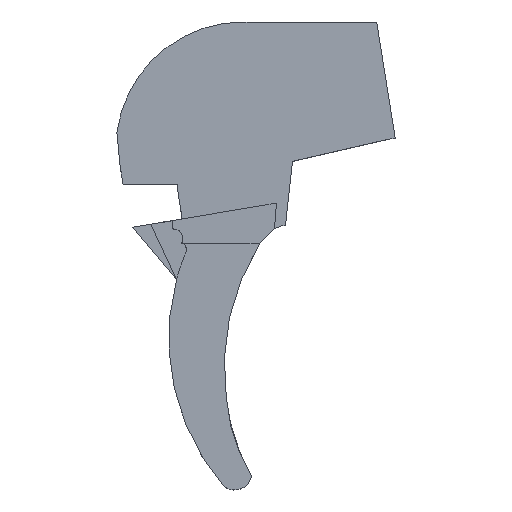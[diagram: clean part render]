
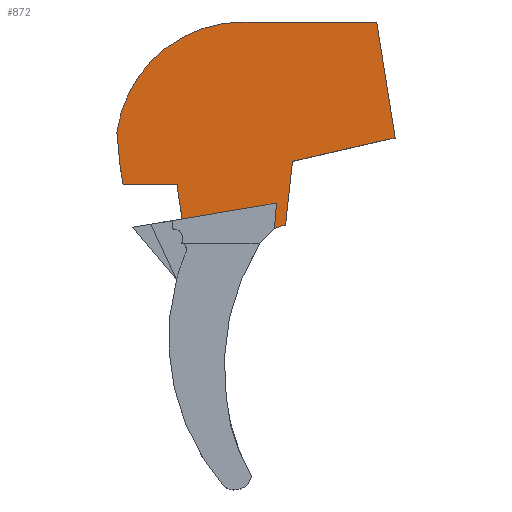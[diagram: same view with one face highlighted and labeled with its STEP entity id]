
A CAD part, top view. The second image highlights one B-rep face of the part: STEP entity #872.
In plain terms, the highlighted planar face has unit normal (0, 0, 1).
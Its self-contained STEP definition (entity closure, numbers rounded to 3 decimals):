
#65=PLANE('',#943);
#100=FACE_OUTER_BOUND('',#148,.T.);
#148=EDGE_LOOP('',(#631,#632,#633,#634,#635,#636,#637,#638,#639,#640,#641,
#642,#643,#644,#645,#646,#647));
#195=LINE('',#1198,#273);
#201=LINE('',#1215,#279);
#218=LINE('',#1272,#296);
#219=LINE('',#1274,#297);
#220=LINE('',#1276,#298);
#221=LINE('',#1277,#299);
#222=LINE('',#1279,#300);
#223=LINE('',#1281,#301);
#224=LINE('',#1283,#302);
#225=LINE('',#1285,#303);
#226=LINE('',#1287,#304);
#227=LINE('',#1289,#305);
#228=LINE('',#1291,#306);
#229=LINE('',#1293,#307);
#230=LINE('',#1294,#308);
#273=VECTOR('',#1000,10.);
#279=VECTOR('',#1014,10.);
#296=VECTOR('',#1045,10.);
#297=VECTOR('',#1046,10.);
#298=VECTOR('',#1047,10.);
#299=VECTOR('',#1048,10.);
#300=VECTOR('',#1049,10.);
#301=VECTOR('',#1050,10.);
#302=VECTOR('',#1051,10.);
#303=VECTOR('',#1052,10.);
#304=VECTOR('',#1053,10.);
#305=VECTOR('',#1054,10.);
#306=VECTOR('',#1055,10.);
#307=VECTOR('',#1056,10.);
#308=VECTOR('',#1057,10.);
#349=CIRCLE('',#930,12.007);
#352=CIRCLE('',#935,3.);
#365=VERTEX_POINT('',#1188);
#366=VERTEX_POINT('',#1189);
#369=VERTEX_POINT('',#1197);
#372=VERTEX_POINT('',#1205);
#375=VERTEX_POINT('',#1212);
#376=VERTEX_POINT('',#1214);
#397=VERTEX_POINT('',#1271);
#398=VERTEX_POINT('',#1273);
#399=VERTEX_POINT('',#1275);
#400=VERTEX_POINT('',#1278);
#401=VERTEX_POINT('',#1280);
#402=VERTEX_POINT('',#1282);
#403=VERTEX_POINT('',#1284);
#404=VERTEX_POINT('',#1286);
#405=VERTEX_POINT('',#1288);
#406=VERTEX_POINT('',#1290);
#407=VERTEX_POINT('',#1292);
#455=EDGE_CURVE('',#365,#366,#349,.T.);
#459=EDGE_CURVE('',#369,#366,#195,.T.);
#464=EDGE_CURVE('',#372,#369,#352,.T.);
#467=EDGE_CURVE('',#376,#375,#201,.T.);
#491=EDGE_CURVE('',#375,#397,#218,.T.);
#492=EDGE_CURVE('',#397,#398,#219,.T.);
#493=EDGE_CURVE('',#398,#399,#220,.T.);
#494=EDGE_CURVE('',#399,#365,#221,.T.);
#495=EDGE_CURVE('',#372,#400,#222,.T.);
#496=EDGE_CURVE('',#400,#401,#223,.T.);
#497=EDGE_CURVE('',#401,#402,#224,.T.);
#498=EDGE_CURVE('',#402,#403,#225,.T.);
#499=EDGE_CURVE('',#404,#403,#226,.T.);
#500=EDGE_CURVE('',#405,#404,#227,.T.);
#501=EDGE_CURVE('',#406,#405,#228,.T.);
#502=EDGE_CURVE('',#406,#407,#229,.T.);
#503=EDGE_CURVE('',#407,#376,#230,.T.);
#631=ORIENTED_EDGE('',*,*,#467,.T.);
#632=ORIENTED_EDGE('',*,*,#491,.T.);
#633=ORIENTED_EDGE('',*,*,#492,.T.);
#634=ORIENTED_EDGE('',*,*,#493,.T.);
#635=ORIENTED_EDGE('',*,*,#494,.T.);
#636=ORIENTED_EDGE('',*,*,#455,.T.);
#637=ORIENTED_EDGE('',*,*,#459,.F.);
#638=ORIENTED_EDGE('',*,*,#464,.F.);
#639=ORIENTED_EDGE('',*,*,#495,.T.);
#640=ORIENTED_EDGE('',*,*,#496,.T.);
#641=ORIENTED_EDGE('',*,*,#497,.T.);
#642=ORIENTED_EDGE('',*,*,#498,.T.);
#643=ORIENTED_EDGE('',*,*,#499,.F.);
#644=ORIENTED_EDGE('',*,*,#500,.F.);
#645=ORIENTED_EDGE('',*,*,#501,.F.);
#646=ORIENTED_EDGE('',*,*,#502,.T.);
#647=ORIENTED_EDGE('',*,*,#503,.T.);
#872=ADVANCED_FACE('',(#100),#65,.T.);
#930=AXIS2_PLACEMENT_3D('',#1190,#992,#993);
#935=AXIS2_PLACEMENT_3D('',#1207,#1008,#1009);
#943=AXIS2_PLACEMENT_3D('',#1270,#1043,#1044);
#992=DIRECTION('center_axis',(0.,0.,
1.));
#993=DIRECTION('ref_axis',(0.,1.,0.));
#1000=DIRECTION('',(-0.094,0.996,0.));
#1008=DIRECTION('center_axis',(0.,0.,
-1.));
#1009=DIRECTION('ref_axis',(-0.809,0.588,0.));
#1014=DIRECTION('',(0.108,0.994,0.));
#1043=DIRECTION('center_axis',(0.,0.,
1.));
#1044=DIRECTION('ref_axis',(0.988,0.156,0.));
#1045=DIRECTION('',(0.975,0.224,0.));
#1046=DIRECTION('',(0.982,0.191,0.));
#1047=DIRECTION('',(-0.156,0.988,0.));
#1048=DIRECTION('',(-1.,0.,0.));
#1049=DIRECTION('',(0.156,-0.988,0.));
#1050=DIRECTION('',(1.,0.,0.));
#1051=DIRECTION('',(0.,-1.,0.));
#1052=DIRECTION('',(0.156,-0.988,0.));
#1053=DIRECTION('',(-0.986,-0.166,0.));
#1054=DIRECTION('',(-0.986,-0.166,0.));
#1055=DIRECTION('',(0.078,0.997,0.));
#1056=DIRECTION('',(0.928,0.373,0.));
#1057=DIRECTION('',(1.,0.,0.));
#1188=CARTESIAN_POINT('',(42.355,145.835,-19.588));
#1189=CARTESIAN_POINT('',(30.449,135.386,-19.588));
#1190=CARTESIAN_POINT('Origin',(42.355,133.828,-19.588));
#1197=CARTESIAN_POINT('',(30.716,132.546,-19.588));
#1198=CARTESIAN_POINT('',(30.539,134.435,-19.588));
#1205=CARTESIAN_POINT('',(30.74,132.357,-19.588));
#1207=CARTESIAN_POINT('Origin',(33.703,132.827,-19.588));
#1212=CARTESIAN_POINT('',(47.029,132.678,-19.588));
#1214=CARTESIAN_POINT('',(46.365,126.592,-19.588));
#1215=CARTESIAN_POINT('',(46.068,123.864,-19.588));
#1270=CARTESIAN_POINT('Origin',(49.799,120.695,-19.588));
#1271=CARTESIAN_POINT('',(56.12,134.767,-19.588));
#1272=CARTESIAN_POINT('',(36.148,130.176,-19.588));
#1273=CARTESIAN_POINT('',(56.719,134.884,-19.588));
#1274=CARTESIAN_POINT('',(56.12,134.767,-19.588));
#1275=CARTESIAN_POINT('',(54.985,145.835,-19.588));
#1276=CARTESIAN_POINT('',(56.719,134.884,-19.588));
#1277=CARTESIAN_POINT('',(54.985,145.835,-19.588));
#1278=CARTESIAN_POINT('',(31.033,130.509,-19.588));
#1279=CARTESIAN_POINT('',(30.271,135.32,-19.588));
#1280=CARTESIAN_POINT('',(36.162,130.509,-19.588));
#1281=CARTESIAN_POINT('',(42.581,130.509,-19.588));
#1282=CARTESIAN_POINT('',(36.162,130.084,-19.588));
#1283=CARTESIAN_POINT('',(36.162,124.802,-19.588));
#1284=CARTESIAN_POINT('',(36.612,127.243,-19.588));
#1285=CARTESIAN_POINT('',(36.148,130.176,-19.588));
#1286=CARTESIAN_POINT('',(44.407,128.557,-19.588));
#1287=CARTESIAN_POINT('',(-34.253,115.292,-19.588));
#1288=CARTESIAN_POINT('',(45.517,128.745,-19.588));
#1289=CARTESIAN_POINT('',(-34.253,115.292,-19.588));
#1290=CARTESIAN_POINT('',(45.329,126.322,-19.588));
#1291=CARTESIAN_POINT('',(43.86,107.439,-19.588));
#1292=CARTESIAN_POINT('',(46.,126.592,-19.588));
#1293=CARTESIAN_POINT('',(45.329,126.322,-19.588));
#1294=CARTESIAN_POINT('',(46.,126.592,-19.588));
